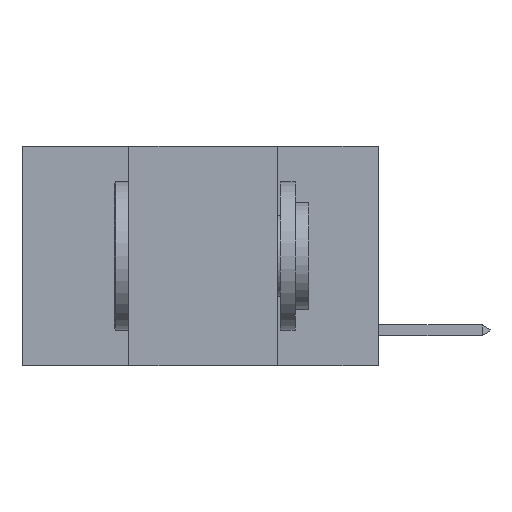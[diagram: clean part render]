
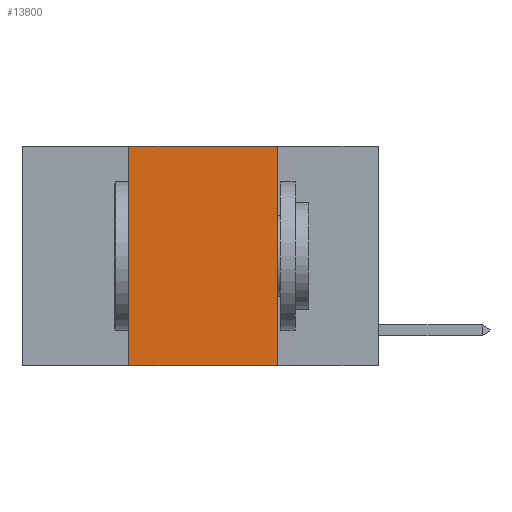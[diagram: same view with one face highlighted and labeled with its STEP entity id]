
A CAD part, left-side view. The second image highlights one B-rep face of the part: STEP entity #13800.
In plain terms, the highlighted planar face has unit normal (-1, 0, 0).
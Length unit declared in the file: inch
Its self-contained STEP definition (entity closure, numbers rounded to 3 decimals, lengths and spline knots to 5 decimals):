
#474 = CARTESIAN_POINT ( 'NONE',  ( 0., 0.6, -0.37 ) ) ;
#812 = LINE ( 'NONE', #8170, #1311 ) ;
#1158 = ORIENTED_EDGE ( 'NONE', *, *, #4270, .F. ) ;
#1311 = VECTOR ( 'NONE', #1786, 39.37008 ) ;
#1786 = DIRECTION ( 'NONE',  ( 0., 0., -1. ) ) ;
#2020 = CARTESIAN_POINT ( 'NONE',  ( 0., 0.42, 0. ) ) ;
#2310 = FACE_OUTER_BOUND ( 'NONE', #10123, .T. ) ;
#2483 = CARTESIAN_POINT ( 'NONE',  ( 0., 0.6, 0. ) ) ;
#3242 = DIRECTION ( 'NONE',  ( 0., 0., 1. ) ) ;
#3494 = VERTEX_POINT ( 'NONE', #14050 ) ;
#4270 = EDGE_CURVE ( 'NONE', #3494, #5557, #812, .T. ) ;
#5557 = VERTEX_POINT ( 'NONE', #8521 ) ;
#5732 = CARTESIAN_POINT ( 'NONE',  ( 0., 0.42, 0. ) ) ;
#5876 = VECTOR ( 'NONE', #8174, 39.37008 ) ;
#6049 = EDGE_CURVE ( 'NONE', #6771, #7006, #9061, .T. ) ;
#6690 = EDGE_CURVE ( 'NONE', #6771, #5557, #8541, .T. ) ;
#6771 = VERTEX_POINT ( 'NONE', #9168 ) ;
#6982 = VECTOR ( 'NONE', #3242, 39.37008 ) ;
#7006 = VERTEX_POINT ( 'NONE', #5732 ) ;
#7139 = ORIENTED_EDGE ( 'NONE', *, *, #6049, .F. ) ;
#7587 = DIRECTION ( 'NONE',  ( 1., 0., 0. ) ) ;
#7722 = DIRECTION ( 'NONE',  ( 0., 0., -1. ) ) ;
#8170 = CARTESIAN_POINT ( 'NONE',  ( 0., 0.17, 0. ) ) ;
#8174 = DIRECTION ( 'NONE',  ( 0., -1., 0. ) ) ;
#8521 = CARTESIAN_POINT ( 'NONE',  ( 0., 0.17, -0.37 ) ) ;
#8541 = LINE ( 'NONE', #474, #11083 ) ;
#9061 = LINE ( 'NONE', #2020, #6982 ) ;
#9168 = CARTESIAN_POINT ( 'NONE',  ( 0., 0.42, -0.37 ) ) ;
#10123 = EDGE_LOOP ( 'NONE', ( #1158, #12191, #7139, #10586 ) ) ;
#10468 = AXIS2_PLACEMENT_3D ( 'NONE', #11883, #7587, #7722 ) ;
#10586 = ORIENTED_EDGE ( 'NONE', *, *, #6690, .T. ) ;
#11043 = LINE ( 'NONE', #2483, #5876 ) ;
#11083 = VECTOR ( 'NONE', #13738, 39.37008 ) ;
#11488 = EDGE_CURVE ( 'NONE', #7006, #3494, #11043, .T. ) ;
#11883 = CARTESIAN_POINT ( 'NONE',  ( 0., 0.6, 0. ) ) ;
#12191 = ORIENTED_EDGE ( 'NONE', *, *, #11488, .F. ) ;
#13738 = DIRECTION ( 'NONE',  ( 0., -1., 0. ) ) ;
#13800 = ADVANCED_FACE ( 'NONE', ( #2310 ), #14301, .F. ) ;
#14050 = CARTESIAN_POINT ( 'NONE',  ( 0., 0.17, 0. ) ) ;
#14301 = PLANE ( 'NONE',  #10468 ) ;
